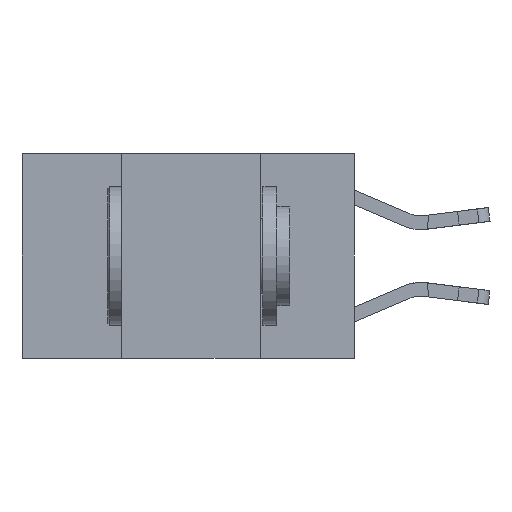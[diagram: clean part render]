
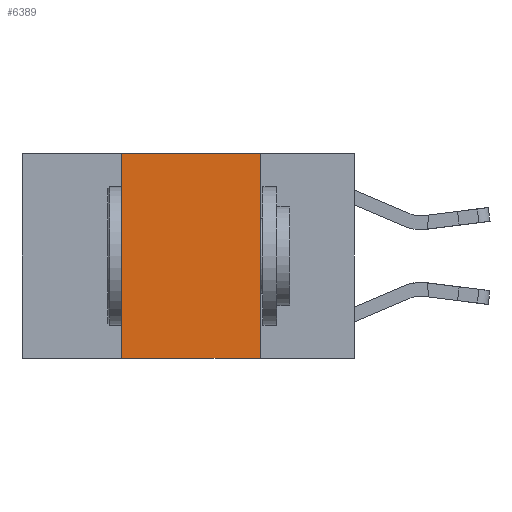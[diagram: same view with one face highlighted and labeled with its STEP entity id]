
A CAD part, left-side view. The second image highlights one B-rep face of the part: STEP entity #6389.
In plain terms, the highlighted planar face has unit normal (-1, 0, 0).
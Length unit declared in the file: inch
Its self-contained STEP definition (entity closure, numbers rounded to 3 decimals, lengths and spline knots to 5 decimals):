
#221 = LINE ( 'NONE', #1712, #9994 ) ;
#791 = CARTESIAN_POINT ( 'NONE',  ( 0., 0.17, 0. ) ) ;
#1163 = VECTOR ( 'NONE', #4666, 39.37008 ) ;
#1712 = CARTESIAN_POINT ( 'NONE',  ( 0., 0.42, 0. ) ) ;
#1977 = LINE ( 'NONE', #791, #5517 ) ;
#2060 = LINE ( 'NONE', #17182, #12103 ) ;
#2262 = CARTESIAN_POINT ( 'NONE',  ( 0., 0.42, -0.37 ) ) ;
#2271 = EDGE_CURVE ( 'NONE', #11735, #16779, #9166, .T. ) ;
#3093 = ORIENTED_EDGE ( 'NONE', *, *, #2271, .F. ) ;
#3547 = PLANE ( 'NONE',  #4200 ) ;
#4200 = AXIS2_PLACEMENT_3D ( 'NONE', #15283, #4840, #12500 ) ;
#4666 = DIRECTION ( 'NONE',  ( 0., -1., 0. ) ) ;
#4840 = DIRECTION ( 'NONE',  ( 1., 0., 0. ) ) ;
#5370 = VERTEX_POINT ( 'NONE', #2262 ) ;
#5517 = VECTOR ( 'NONE', #8471, 39.37008 ) ;
#6389 = ADVANCED_FACE ( 'NONE', ( #18461 ), #3547, .F. ) ;
#6638 = ORIENTED_EDGE ( 'NONE', *, *, #8748, .F. ) ;
#7671 = CARTESIAN_POINT ( 'NONE',  ( 0., 0.6, 0. ) ) ;
#8471 = DIRECTION ( 'NONE',  ( 0., 0., -1. ) ) ;
#8656 = ORIENTED_EDGE ( 'NONE', *, *, #11029, .T. ) ;
#8662 = CARTESIAN_POINT ( 'NONE',  ( 0., 0.17, -0.37 ) ) ;
#8748 = EDGE_CURVE ( 'NONE', #5370, #11735, #221, .T. ) ;
#9166 = LINE ( 'NONE', #7671, #1163 ) ;
#9346 = EDGE_CURVE ( 'NONE', #16779, #9551, #1977, .T. ) ;
#9551 = VERTEX_POINT ( 'NONE', #8662 ) ;
#9994 = VECTOR ( 'NONE', #16830, 39.37008 ) ;
#10160 = EDGE_LOOP ( 'NONE', ( #10745, #3093, #6638, #8656 ) ) ;
#10745 = ORIENTED_EDGE ( 'NONE', *, *, #9346, .F. ) ;
#11029 = EDGE_CURVE ( 'NONE', #5370, #9551, #2060, .T. ) ;
#11735 = VERTEX_POINT ( 'NONE', #18222 ) ;
#12103 = VECTOR ( 'NONE', #14100, 39.37008 ) ;
#12500 = DIRECTION ( 'NONE',  ( 0., 0., -1. ) ) ;
#14100 = DIRECTION ( 'NONE',  ( 0., -1., 0. ) ) ;
#15283 = CARTESIAN_POINT ( 'NONE',  ( 0., 0.6, 0. ) ) ;
#16444 = CARTESIAN_POINT ( 'NONE',  ( 0., 0.17, 0. ) ) ;
#16779 = VERTEX_POINT ( 'NONE', #16444 ) ;
#16830 = DIRECTION ( 'NONE',  ( 0., 0., 1. ) ) ;
#17182 = CARTESIAN_POINT ( 'NONE',  ( 0., 0.6, -0.37 ) ) ;
#18222 = CARTESIAN_POINT ( 'NONE',  ( 0., 0.42, 0. ) ) ;
#18461 = FACE_OUTER_BOUND ( 'NONE', #10160, .T. ) ;
